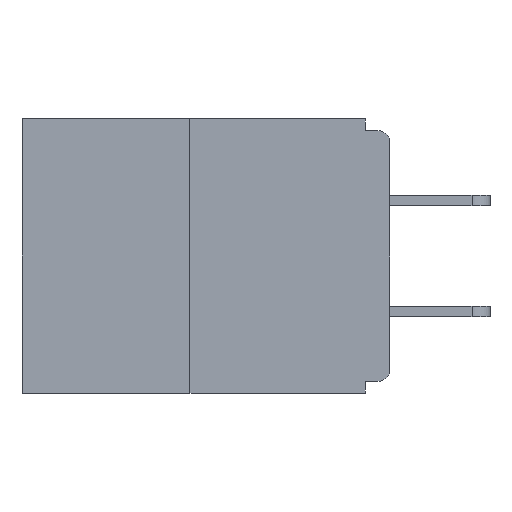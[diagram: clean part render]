
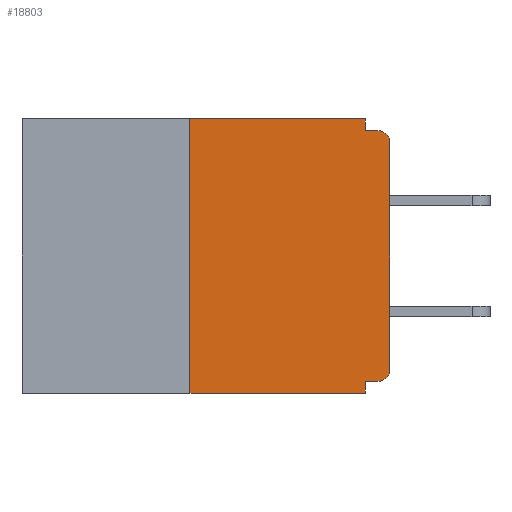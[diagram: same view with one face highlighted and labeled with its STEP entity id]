
A CAD part, left-side view. The second image highlights one B-rep face of the part: STEP entity #18803.
In plain terms, the highlighted planar face has unit normal (-1, 0, 0).
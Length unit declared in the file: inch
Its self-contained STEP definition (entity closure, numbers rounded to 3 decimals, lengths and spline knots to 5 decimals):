
#410 = DIRECTION ( 'NONE',  ( 0., 1., 0. ) ) ;
#750 = CARTESIAN_POINT ( 'NONE',  ( 0., 0.25, 0. ) ) ;
#925 = CARTESIAN_POINT ( 'NONE',  ( 0., 0., -0.015 ) ) ;
#1003 = VERTEX_POINT ( 'NONE', #12629 ) ;
#1491 = CIRCLE ( 'NONE', #10321, 0.015 ) ;
#1729 = CARTESIAN_POINT ( 'NONE',  ( 0., 0.46, 0. ) ) ;
#1883 = LINE ( 'NONE', #19859, #7733 ) ;
#2185 = VECTOR ( 'NONE', #22420, 39.37008 ) ;
#2593 = ORIENTED_EDGE ( 'NONE', *, *, #17401, .T. ) ;
#2655 = DIRECTION ( 'NONE',  ( 0., -1., 0. ) ) ;
#3316 = ORIENTED_EDGE ( 'NONE', *, *, #20832, .F. ) ;
#3767 = CARTESIAN_POINT ( 'NONE',  ( 0., 0.46, 0. ) ) ;
#3983 = EDGE_CURVE ( 'NONE', #19490, #24828, #1491, .T. ) ;
#4748 = LINE ( 'NONE', #6777, #24978 ) ;
#5084 = ORIENTED_EDGE ( 'NONE', *, *, #11963, .F. ) ;
#5513 = CARTESIAN_POINT ( 'NONE',  ( 0., 0.015, -0.313 ) ) ;
#5598 = CARTESIAN_POINT ( 'NONE',  ( 0., 0.031, 0. ) ) ;
#5906 = DIRECTION ( 'NONE',  ( 0., -1., 0. ) ) ;
#5937 = VERTEX_POINT ( 'NONE', #17418 ) ;
#6410 = EDGE_CURVE ( 'NONE', #5937, #24828, #21658, .T. ) ;
#6437 = EDGE_CURVE ( 'NONE', #18816, #24362, #4748, .T. ) ;
#6777 = CARTESIAN_POINT ( 'NONE',  ( 0., 0.46, -0.343 ) ) ;
#7067 = CARTESIAN_POINT ( 'NONE',  ( 0., 0.031, -0.343 ) ) ;
#7154 = CARTESIAN_POINT ( 'NONE',  ( 0., 0., -0.03 ) ) ;
#7733 = VECTOR ( 'NONE', #13689, 39.37008 ) ;
#7838 = ORIENTED_EDGE ( 'NONE', *, *, #21858, .F. ) ;
#8148 = VECTOR ( 'NONE', #24106, 39.37008 ) ;
#8566 = DIRECTION ( 'NONE',  ( 0., -1., 0. ) ) ;
#9015 = CARTESIAN_POINT ( 'NONE',  ( 0., 0., 0. ) ) ;
#9308 = AXIS2_PLACEMENT_3D ( 'NONE', #1729, #15479, #13937 ) ;
#9670 = LINE ( 'NONE', #750, #17391 ) ;
#9984 = VECTOR ( 'NONE', #2655, 39.37008 ) ;
#10268 = LINE ( 'NONE', #16147, #8148 ) ;
#10321 = AXIS2_PLACEMENT_3D ( 'NONE', #15488, #17297, #21254 ) ;
#11264 = AXIS2_PLACEMENT_3D ( 'NONE', #5513, #19249, #20960 ) ;
#11670 = ORIENTED_EDGE ( 'NONE', *, *, #12002, .F. ) ;
#11860 = CARTESIAN_POINT ( 'NONE',  ( 0., 0.015, -0.328 ) ) ;
#11963 = EDGE_CURVE ( 'NONE', #18816, #1003, #9670, .T. ) ;
#12002 = EDGE_CURVE ( 'NONE', #21850, #24362, #10268, .T. ) ;
#12173 = CARTESIAN_POINT ( 'NONE',  ( 0., 0., -0.328 ) ) ;
#12629 = CARTESIAN_POINT ( 'NONE',  ( 0., 0.25, 0. ) ) ;
#12688 = VERTEX_POINT ( 'NONE', #11860 ) ;
#13689 = DIRECTION ( 'NONE',  ( 0., 0., -1. ) ) ;
#13859 = CARTESIAN_POINT ( 'NONE',  ( 0., 0.25, -0.343 ) ) ;
#13937 = DIRECTION ( 'NONE',  ( 0., 0., -1. ) ) ;
#14612 = VECTOR ( 'NONE', #410, 39.37008 ) ;
#15479 = DIRECTION ( 'NONE',  ( 1., 0., 0. ) ) ;
#15483 = VERTEX_POINT ( 'NONE', #25309 ) ;
#15488 = CARTESIAN_POINT ( 'NONE',  ( 0., 0.015, -0.03 ) ) ;
#15566 = CIRCLE ( 'NONE', #11264, 0.015 ) ;
#15928 = VECTOR ( 'NONE', #5906, 39.37008 ) ;
#16147 = CARTESIAN_POINT ( 'NONE',  ( 0., 0.031, -0.343 ) ) ;
#16234 = DIRECTION ( 'NONE',  ( 0., 0., 1. ) ) ;
#16751 = CARTESIAN_POINT ( 'NONE',  ( 0., 0.015, -0.015 ) ) ;
#17297 = DIRECTION ( 'NONE',  ( -1., 0., 0. ) ) ;
#17391 = VECTOR ( 'NONE', #16234, 39.37008 ) ;
#17396 = LINE ( 'NONE', #12173, #14612 ) ;
#17401 = EDGE_CURVE ( 'NONE', #12688, #15483, #15566, .T. ) ;
#17418 = CARTESIAN_POINT ( 'NONE',  ( 0., 0.031, -0.015 ) ) ;
#18769 = ORIENTED_EDGE ( 'NONE', *, *, #3983, .T. ) ;
#18803 = ADVANCED_FACE ( 'NONE', ( #19496 ), #23701, .F. ) ;
#18816 = VERTEX_POINT ( 'NONE', #13859 ) ;
#19249 = DIRECTION ( 'NONE',  ( -1., 0., 0. ) ) ;
#19490 = VERTEX_POINT ( 'NONE', #7154 ) ;
#19496 = FACE_OUTER_BOUND ( 'NONE', #22868, .T. ) ;
#19859 = CARTESIAN_POINT ( 'NONE',  ( 0., 0.031, 0. ) ) ;
#20005 = LINE ( 'NONE', #9015, #2185 ) ;
#20429 = EDGE_CURVE ( 'NONE', #15483, #19490, #20005, .T. ) ;
#20832 = EDGE_CURVE ( 'NONE', #22629, #5937, #1883, .T. ) ;
#20960 = DIRECTION ( 'NONE',  ( 0., 0., -1. ) ) ;
#21254 = DIRECTION ( 'NONE',  ( 0., 0., -1. ) ) ;
#21658 = LINE ( 'NONE', #925, #9984 ) ;
#21850 = VERTEX_POINT ( 'NONE', #23577 ) ;
#21858 = EDGE_CURVE ( 'NONE', #1003, #22629, #23891, .T. ) ;
#22073 = ORIENTED_EDGE ( 'NONE', *, *, #20429, .T. ) ;
#22420 = DIRECTION ( 'NONE',  ( 0., 0., 1. ) ) ;
#22629 = VERTEX_POINT ( 'NONE', #5598 ) ;
#22868 = EDGE_LOOP ( 'NONE', ( #7838, #5084, #23002, #11670, #25047, #2593, #22073, #18769, #23406, #3316 ) ) ;
#23002 = ORIENTED_EDGE ( 'NONE', *, *, #6437, .T. ) ;
#23274 = EDGE_CURVE ( 'NONE', #12688, #21850, #17396, .T. ) ;
#23406 = ORIENTED_EDGE ( 'NONE', *, *, #6410, .F. ) ;
#23577 = CARTESIAN_POINT ( 'NONE',  ( 0., 0.031, -0.328 ) ) ;
#23701 = PLANE ( 'NONE',  #9308 ) ;
#23891 = LINE ( 'NONE', #3767, #15928 ) ;
#24106 = DIRECTION ( 'NONE',  ( 0., 0., -1. ) ) ;
#24362 = VERTEX_POINT ( 'NONE', #7067 ) ;
#24828 = VERTEX_POINT ( 'NONE', #16751 ) ;
#24978 = VECTOR ( 'NONE', #8566, 39.37008 ) ;
#25047 = ORIENTED_EDGE ( 'NONE', *, *, #23274, .F. ) ;
#25309 = CARTESIAN_POINT ( 'NONE',  ( 0., 0., -0.313 ) ) ;
